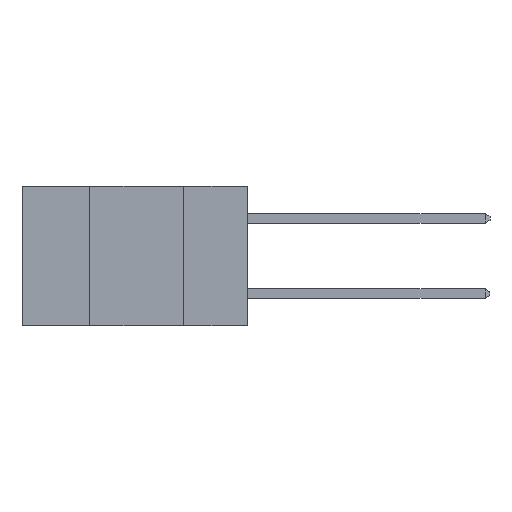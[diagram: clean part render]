
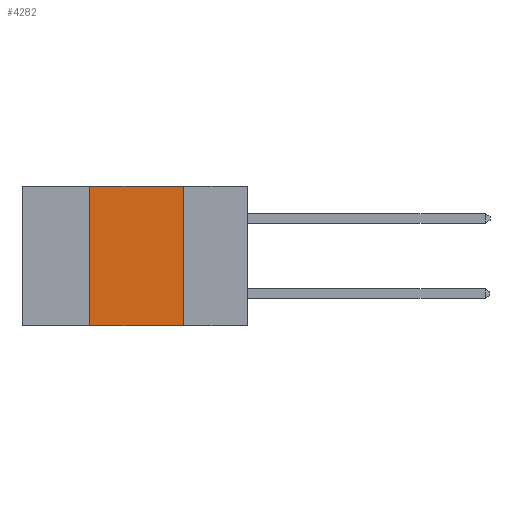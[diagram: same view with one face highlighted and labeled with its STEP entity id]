
A CAD part, left-side view. The second image highlights one B-rep face of the part: STEP entity #4282.
In plain terms, the highlighted planar face has unit normal (-1, 0, 0).
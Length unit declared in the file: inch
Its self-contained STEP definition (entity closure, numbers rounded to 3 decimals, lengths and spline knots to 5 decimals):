
#554 = VERTEX_POINT ( 'NONE', #21779 ) ;
#1244 = ORIENTED_EDGE ( 'NONE', *, *, #4011, .T. ) ;
#3623 = CARTESIAN_POINT ( 'NONE',  ( 0., 0.42, 0. ) ) ;
#4011 = EDGE_CURVE ( 'NONE', #5516, #11223, #4618, .T. ) ;
#4282 = ADVANCED_FACE ( 'NONE', ( #11696 ), #23373, .F. ) ;
#4618 = LINE ( 'NONE', #24451, #14982 ) ;
#5516 = VERTEX_POINT ( 'NONE', #17588 ) ;
#6648 = CARTESIAN_POINT ( 'NONE',  ( 0., 0.17, 0. ) ) ;
#6915 = ORIENTED_EDGE ( 'NONE', *, *, #17367, .F. ) ;
#7696 = CARTESIAN_POINT ( 'NONE',  ( 0., 0.17, -0.37 ) ) ;
#8121 = CARTESIAN_POINT ( 'NONE',  ( 0., 0.6, 0. ) ) ;
#8204 = LINE ( 'NONE', #3623, #22842 ) ;
#11223 = VERTEX_POINT ( 'NONE', #7696 ) ;
#11645 = EDGE_LOOP ( 'NONE', ( #22206, #6915, #24220, #1244 ) ) ;
#11696 = FACE_OUTER_BOUND ( 'NONE', #11645, .T. ) ;
#11952 = DIRECTION ( 'NONE',  ( 1., 0., 0. ) ) ;
#12031 = DIRECTION ( 'NONE',  ( 0., 0., -1. ) ) ;
#12247 = AXIS2_PLACEMENT_3D ( 'NONE', #8121, #11952, #12031 ) ;
#12547 = DIRECTION ( 'NONE',  ( 0., 0., -1. ) ) ;
#13565 = CARTESIAN_POINT ( 'NONE',  ( 0., 0.17, 0. ) ) ;
#14982 = VECTOR ( 'NONE', #15112, 39.37008 ) ;
#15112 = DIRECTION ( 'NONE',  ( 0., -1., 0. ) ) ;
#16151 = EDGE_CURVE ( 'NONE', #20270, #11223, #16470, .T. ) ;
#16470 = LINE ( 'NONE', #6648, #17057 ) ;
#17057 = VECTOR ( 'NONE', #12547, 39.37008 ) ;
#17147 = DIRECTION ( 'NONE',  ( 0., 0., 1. ) ) ;
#17367 = EDGE_CURVE ( 'NONE', #554, #20270, #23419, .T. ) ;
#17396 = EDGE_CURVE ( 'NONE', #5516, #554, #8204, .T. ) ;
#17588 = CARTESIAN_POINT ( 'NONE',  ( 0., 0.42, -0.37 ) ) ;
#18416 = VECTOR ( 'NONE', #20852, 39.37008 ) ;
#18892 = CARTESIAN_POINT ( 'NONE',  ( 0., 0.6, 0. ) ) ;
#20270 = VERTEX_POINT ( 'NONE', #13565 ) ;
#20852 = DIRECTION ( 'NONE',  ( 0., -1., 0. ) ) ;
#21779 = CARTESIAN_POINT ( 'NONE',  ( 0., 0.42, 0. ) ) ;
#22206 = ORIENTED_EDGE ( 'NONE', *, *, #16151, .F. ) ;
#22842 = VECTOR ( 'NONE', #17147, 39.37008 ) ;
#23373 = PLANE ( 'NONE',  #12247 ) ;
#23419 = LINE ( 'NONE', #18892, #18416 ) ;
#24220 = ORIENTED_EDGE ( 'NONE', *, *, #17396, .F. ) ;
#24451 = CARTESIAN_POINT ( 'NONE',  ( 0., 0.6, -0.37 ) ) ;
